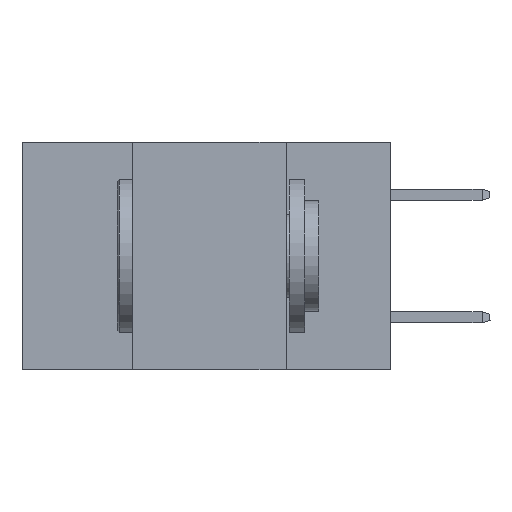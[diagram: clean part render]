
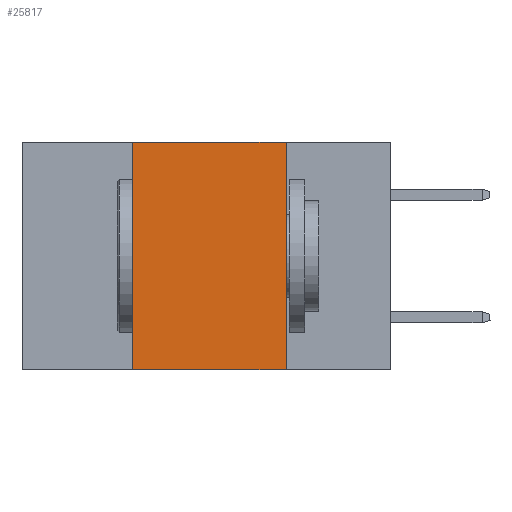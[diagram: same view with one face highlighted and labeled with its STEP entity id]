
A CAD part, left-side view. The second image highlights one B-rep face of the part: STEP entity #25817.
In plain terms, the highlighted planar face has unit normal (-1, 0, 0).
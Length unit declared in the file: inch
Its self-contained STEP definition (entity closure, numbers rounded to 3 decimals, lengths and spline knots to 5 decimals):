
#1000 = DIRECTION ( 'NONE',  ( 0., 0., -1. ) ) ;
#1988 = LINE ( 'NONE', #23414, #6897 ) ;
#2911 = VECTOR ( 'NONE', #1000, 39.37008 ) ;
#3527 = CARTESIAN_POINT ( 'NONE',  ( 0., 0.17, 0. ) ) ;
#5884 = LINE ( 'NONE', #3527, #2911 ) ;
#6124 = EDGE_CURVE ( 'NONE', #21808, #36288, #22239, .T. ) ;
#6469 = EDGE_CURVE ( 'NONE', #21808, #29145, #1988, .T. ) ;
#6897 = VECTOR ( 'NONE', #7760, 39.37008 ) ;
#7760 = DIRECTION ( 'NONE',  ( 0., 0., 1. ) ) ;
#7794 = ORIENTED_EDGE ( 'NONE', *, *, #24249, .F. ) ;
#8581 = ORIENTED_EDGE ( 'NONE', *, *, #6469, .F. ) ;
#9164 = CARTESIAN_POINT ( 'NONE',  ( 0., 0.6, 0. ) ) ;
#12050 = EDGE_CURVE ( 'NONE', #12958, #36288, #5884, .T. ) ;
#12958 = VERTEX_POINT ( 'NONE', #24413 ) ;
#15304 = DIRECTION ( 'NONE',  ( 1., 0., 0. ) ) ;
#15350 = VECTOR ( 'NONE', #39410, 39.37008 ) ;
#20816 = VECTOR ( 'NONE', #34371, 39.37008 ) ;
#21565 = AXIS2_PLACEMENT_3D ( 'NONE', #9164, #15304, #31345 ) ;
#21580 = CARTESIAN_POINT ( 'NONE',  ( 0., 0.42, -0.37 ) ) ;
#21808 = VERTEX_POINT ( 'NONE', #21580 ) ;
#22233 = CARTESIAN_POINT ( 'NONE',  ( 0., 0.17, -0.37 ) ) ;
#22239 = LINE ( 'NONE', #39551, #15350 ) ;
#23414 = CARTESIAN_POINT ( 'NONE',  ( 0., 0.42, 0. ) ) ;
#23534 = CARTESIAN_POINT ( 'NONE',  ( 0., 0.42, 0. ) ) ;
#24249 = EDGE_CURVE ( 'NONE', #29145, #12958, #29200, .T. ) ;
#24413 = CARTESIAN_POINT ( 'NONE',  ( 0., 0.17, 0. ) ) ;
#25817 = ADVANCED_FACE ( 'NONE', ( #27903 ), #34645, .F. ) ;
#27903 = FACE_OUTER_BOUND ( 'NONE', #39073, .T. ) ;
#28805 = ORIENTED_EDGE ( 'NONE', *, *, #12050, .F. ) ;
#29145 = VERTEX_POINT ( 'NONE', #23534 ) ;
#29200 = LINE ( 'NONE', #31223, #20816 ) ;
#31223 = CARTESIAN_POINT ( 'NONE',  ( 0., 0.6, 0. ) ) ;
#31345 = DIRECTION ( 'NONE',  ( 0., 0., -1. ) ) ;
#34371 = DIRECTION ( 'NONE',  ( 0., -1., 0. ) ) ;
#34645 = PLANE ( 'NONE',  #21565 ) ;
#35346 = ORIENTED_EDGE ( 'NONE', *, *, #6124, .T. ) ;
#36288 = VERTEX_POINT ( 'NONE', #22233 ) ;
#39073 = EDGE_LOOP ( 'NONE', ( #28805, #7794, #8581, #35346 ) ) ;
#39410 = DIRECTION ( 'NONE',  ( 0., -1., 0. ) ) ;
#39551 = CARTESIAN_POINT ( 'NONE',  ( 0., 0.6, -0.37 ) ) ;
